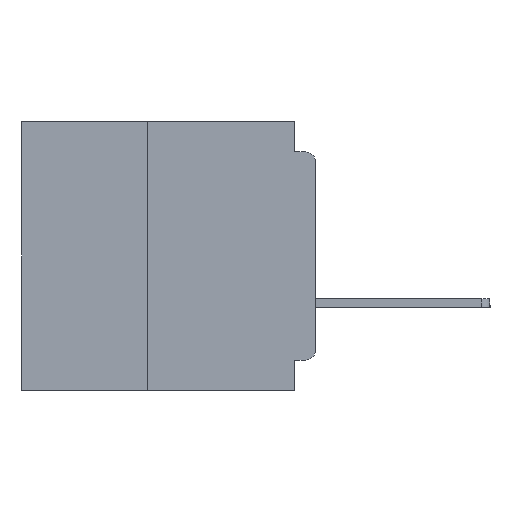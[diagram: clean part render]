
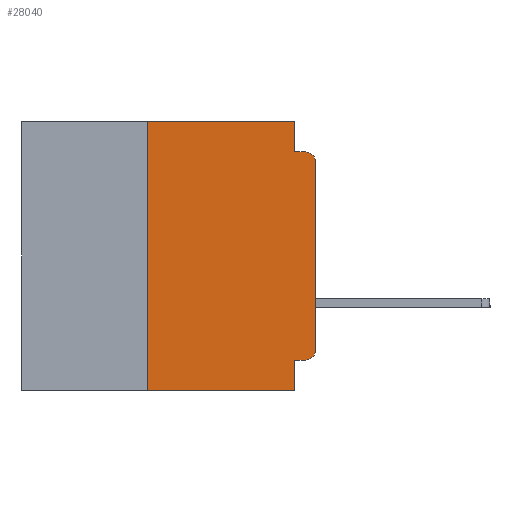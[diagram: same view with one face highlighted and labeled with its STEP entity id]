
A CAD part, left-side view. The second image highlights one B-rep face of the part: STEP entity #28040.
In plain terms, the highlighted planar face has unit normal (-1, 0, 0).
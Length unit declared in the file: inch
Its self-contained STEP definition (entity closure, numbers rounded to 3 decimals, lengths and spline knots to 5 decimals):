
#969 = VERTEX_POINT ( 'NONE', #34587 ) ;
#1188 = CARTESIAN_POINT ( 'NONE',  ( 0., 0.031, -0.4 ) ) ;
#1798 = ORIENTED_EDGE ( 'NONE', *, *, #33661, .T. ) ;
#2278 = VERTEX_POINT ( 'NONE', #26718 ) ;
#3736 = EDGE_CURVE ( 'NONE', #8397, #21009, #5854, .T. ) ;
#3842 = ORIENTED_EDGE ( 'NONE', *, *, #14986, .F. ) ;
#4198 = ORIENTED_EDGE ( 'NONE', *, *, #5563, .F. ) ;
#4507 = LINE ( 'NONE', #28009, #24316 ) ;
#4837 = VERTEX_POINT ( 'NONE', #16845 ) ;
#4863 = VECTOR ( 'NONE', #22117, 39.37008 ) ;
#5010 = VECTOR ( 'NONE', #11218, 39.37008 ) ;
#5314 = AXIS2_PLACEMENT_3D ( 'NONE', #6484, #25336, #9211 ) ;
#5563 = EDGE_CURVE ( 'NONE', #32710, #11878, #4507, .T. ) ;
#5854 = LINE ( 'NONE', #33935, #5010 ) ;
#5860 = CARTESIAN_POINT ( 'NONE',  ( 0., 0., 0. ) ) ;
#6273 = LINE ( 'NONE', #33779, #20584 ) ;
#6484 = CARTESIAN_POINT ( 'NONE',  ( 0., 0.015, -0.06 ) ) ;
#7294 = VERTEX_POINT ( 'NONE', #30092 ) ;
#7779 = ORIENTED_EDGE ( 'NONE', *, *, #22554, .T. ) ;
#8320 = FACE_OUTER_BOUND ( 'NONE', #8324, .T. ) ;
#8324 = EDGE_LOOP ( 'NONE', ( #22879, #7779, #20439, #4198, #21500, #24212, #1798, #3842, #8464, #18919 ) ) ;
#8397 = VERTEX_POINT ( 'NONE', #23279 ) ;
#8464 = ORIENTED_EDGE ( 'NONE', *, *, #3736, .F. ) ;
#8581 = DIRECTION ( 'NONE',  ( 0., 0., 1. ) ) ;
#9211 = DIRECTION ( 'NONE',  ( 0., 0., -1. ) ) ;
#10385 = CARTESIAN_POINT ( 'NONE',  ( 0., 0.031, 0. ) ) ;
#11218 = DIRECTION ( 'NONE',  ( 0., 1., 0. ) ) ;
#11733 = CARTESIAN_POINT ( 'NONE',  ( 0., 0.437, -0.4 ) ) ;
#11878 = VERTEX_POINT ( 'NONE', #33015 ) ;
#11971 = DIRECTION ( 'NONE',  ( 1., 0., 0. ) ) ;
#12705 = EDGE_CURVE ( 'NONE', #25719, #7294, #28934, .T. ) ;
#12887 = VERTEX_POINT ( 'NONE', #30791 ) ;
#14438 = DIRECTION ( 'NONE',  ( -1., 0., 0. ) ) ;
#14986 = EDGE_CURVE ( 'NONE', #21009, #4837, #28061, .T. ) ;
#15465 = EDGE_CURVE ( 'NONE', #11878, #2278, #19199, .T. ) ;
#15654 = CARTESIAN_POINT ( 'NONE',  ( 0., 0.031, -0.355 ) ) ;
#16072 = VECTOR ( 'NONE', #31672, 39.37008 ) ;
#16845 = CARTESIAN_POINT ( 'NONE',  ( 0., 0.031, -0.4 ) ) ;
#16918 = LINE ( 'NONE', #23542, #16072 ) ;
#17652 = DIRECTION ( 'NONE',  ( 0., -1., 0. ) ) ;
#18391 = LINE ( 'NONE', #11733, #24748 ) ;
#18919 = ORIENTED_EDGE ( 'NONE', *, *, #20051, .T. ) ;
#19199 = LINE ( 'NONE', #24842, #4863 ) ;
#20051 = EDGE_CURVE ( 'NONE', #8397, #25719, #27683, .T. ) ;
#20439 = ORIENTED_EDGE ( 'NONE', *, *, #15465, .F. ) ;
#20584 = VECTOR ( 'NONE', #17652, 39.37008 ) ;
#20908 = VECTOR ( 'NONE', #25456, 39.37008 ) ;
#21009 = VERTEX_POINT ( 'NONE', #15654 ) ;
#21500 = ORIENTED_EDGE ( 'NONE', *, *, #32556, .F. ) ;
#21759 = VECTOR ( 'NONE', #8581, 39.37008 ) ;
#22117 = DIRECTION ( 'NONE',  ( 0., -1., 0. ) ) ;
#22554 = EDGE_CURVE ( 'NONE', #7294, #2278, #23696, .T. ) ;
#22804 = EDGE_CURVE ( 'NONE', #969, #12887, #16918, .T. ) ;
#22879 = ORIENTED_EDGE ( 'NONE', *, *, #12705, .T. ) ;
#23279 = CARTESIAN_POINT ( 'NONE',  ( 0., 0.015, -0.355 ) ) ;
#23542 = CARTESIAN_POINT ( 'NONE',  ( 0., 0.25, -0.4 ) ) ;
#23696 = CIRCLE ( 'NONE', #5314, 0.015 ) ;
#24212 = ORIENTED_EDGE ( 'NONE', *, *, #22804, .F. ) ;
#24316 = VECTOR ( 'NONE', #28031, 39.37008 ) ;
#24475 = AXIS2_PLACEMENT_3D ( 'NONE', #28080, #11971, #30787 ) ;
#24748 = VECTOR ( 'NONE', #33251, 39.37008 ) ;
#24842 = CARTESIAN_POINT ( 'NONE',  ( 0., 0., -0.045 ) ) ;
#25336 = DIRECTION ( 'NONE',  ( -1., 0., 0. ) ) ;
#25394 = PLANE ( 'NONE',  #24475 ) ;
#25456 = DIRECTION ( 'NONE',  ( 0., 0., -1. ) ) ;
#25719 = VERTEX_POINT ( 'NONE', #29789 ) ;
#26718 = CARTESIAN_POINT ( 'NONE',  ( 0., 0.015, -0.045 ) ) ;
#27683 = CIRCLE ( 'NONE', #33648, 0.015 ) ;
#28009 = CARTESIAN_POINT ( 'NONE',  ( 0., 0.031, 0. ) ) ;
#28031 = DIRECTION ( 'NONE',  ( 0., 0., -1. ) ) ;
#28040 = ADVANCED_FACE ( 'NONE', ( #8320 ), #25394, .F. ) ;
#28061 = LINE ( 'NONE', #1188, #20908 ) ;
#28080 = CARTESIAN_POINT ( 'NONE',  ( 0., 0.437, 0. ) ) ;
#28934 = LINE ( 'NONE', #5860, #21759 ) ;
#29789 = CARTESIAN_POINT ( 'NONE',  ( 0., 0., -0.34 ) ) ;
#30092 = CARTESIAN_POINT ( 'NONE',  ( 0., 0., -0.06 ) ) ;
#30553 = CARTESIAN_POINT ( 'NONE',  ( 0., 0.015, -0.34 ) ) ;
#30787 = DIRECTION ( 'NONE',  ( 0., 0., -1. ) ) ;
#30791 = CARTESIAN_POINT ( 'NONE',  ( 0., 0.25, 0. ) ) ;
#31672 = DIRECTION ( 'NONE',  ( 0., 0., 1. ) ) ;
#32556 = EDGE_CURVE ( 'NONE', #12887, #32710, #6273, .T. ) ;
#32710 = VERTEX_POINT ( 'NONE', #10385 ) ;
#33015 = CARTESIAN_POINT ( 'NONE',  ( 0., 0.031, -0.045 ) ) ;
#33251 = DIRECTION ( 'NONE',  ( 0., -1., 0. ) ) ;
#33259 = DIRECTION ( 'NONE',  ( 0., 0., -1. ) ) ;
#33648 = AXIS2_PLACEMENT_3D ( 'NONE', #30553, #14438, #33259 ) ;
#33661 = EDGE_CURVE ( 'NONE', #969, #4837, #18391, .T. ) ;
#33779 = CARTESIAN_POINT ( 'NONE',  ( 0., 0.437, 0. ) ) ;
#33935 = CARTESIAN_POINT ( 'NONE',  ( 0., 0., -0.355 ) ) ;
#34587 = CARTESIAN_POINT ( 'NONE',  ( 0., 0.25, -0.4 ) ) ;
